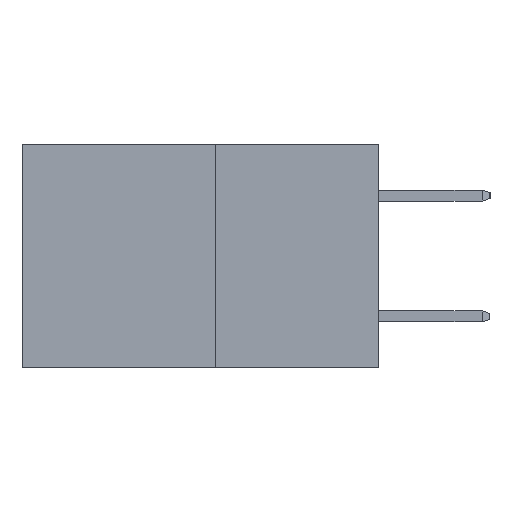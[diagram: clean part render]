
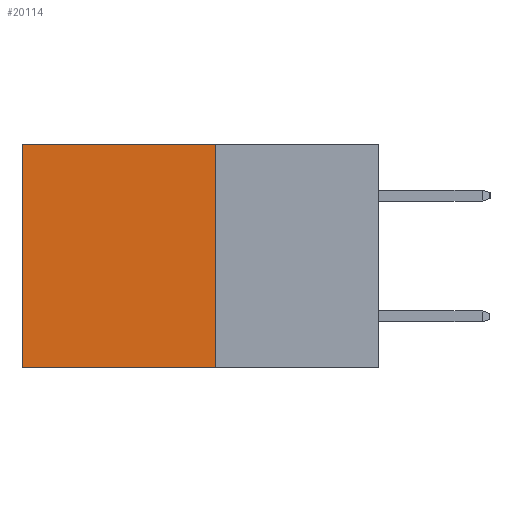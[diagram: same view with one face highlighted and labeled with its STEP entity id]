
A CAD part, left-side view. The second image highlights one B-rep face of the part: STEP entity #20114.
In plain terms, the highlighted planar face has unit normal (-1, 0, 0).
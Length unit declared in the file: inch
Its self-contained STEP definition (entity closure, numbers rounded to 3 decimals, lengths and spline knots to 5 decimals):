
#370 = VECTOR ( 'NONE', #7901, 39.37008 ) ;
#1036 = EDGE_LOOP ( 'NONE', ( #13480, #3146, #9944, #14698 ) ) ;
#1885 = CARTESIAN_POINT ( 'NONE',  ( 0.277, 0.59, -0.37 ) ) ;
#2615 = DIRECTION ( 'NONE',  ( 1., 0., 0. ) ) ;
#3146 = ORIENTED_EDGE ( 'NONE', *, *, #12258, .F. ) ;
#5349 = VERTEX_POINT ( 'NONE', #1885 ) ;
#5377 = LINE ( 'NONE', #17044, #370 ) ;
#5748 = VERTEX_POINT ( 'NONE', #22098 ) ;
#6297 = PLANE ( 'NONE',  #23699 ) ;
#7901 = DIRECTION ( 'NONE',  ( 0., 1., 0. ) ) ;
#8111 = LINE ( 'NONE', #21668, #17305 ) ;
#8784 = CARTESIAN_POINT ( 'NONE',  ( 0.277, 0.27, -0.37 ) ) ;
#8902 = DIRECTION ( 'NONE',  ( 0., 0., -1. ) ) ;
#9064 = VECTOR ( 'NONE', #17220, 39.37008 ) ;
#9944 = ORIENTED_EDGE ( 'NONE', *, *, #23379, .F. ) ;
#10613 = FACE_OUTER_BOUND ( 'NONE', #1036, .T. ) ;
#11585 = DIRECTION ( 'NONE',  ( 0., 0., -1. ) ) ;
#12258 = EDGE_CURVE ( 'NONE', #14520, #5349, #14532, .T. ) ;
#12413 = VERTEX_POINT ( 'NONE', #13936 ) ;
#13480 = ORIENTED_EDGE ( 'NONE', *, *, #14127, .T. ) ;
#13714 = CARTESIAN_POINT ( 'NONE',  ( 0.277, 0.27, -0.37 ) ) ;
#13936 = CARTESIAN_POINT ( 'NONE',  ( 0.277, 0.27, 0. ) ) ;
#14127 = EDGE_CURVE ( 'NONE', #5748, #5349, #21295, .T. ) ;
#14520 = VERTEX_POINT ( 'NONE', #8784 ) ;
#14532 = LINE ( 'NONE', #15400, #9064 ) ;
#14698 = ORIENTED_EDGE ( 'NONE', *, *, #18760, .T. ) ;
#15400 = CARTESIAN_POINT ( 'NONE',  ( 0.277, 0.27, -0.37 ) ) ;
#15565 = DIRECTION ( 'NONE',  ( 0., 0., -1. ) ) ;
#16436 = VECTOR ( 'NONE', #11585, 39.37008 ) ;
#17044 = CARTESIAN_POINT ( 'NONE',  ( 0.277, 0.27, 0. ) ) ;
#17220 = DIRECTION ( 'NONE',  ( 0., 1., 0. ) ) ;
#17305 = VECTOR ( 'NONE', #8902, 39.37008 ) ;
#18760 = EDGE_CURVE ( 'NONE', #12413, #5748, #5377, .T. ) ;
#18819 = CARTESIAN_POINT ( 'NONE',  ( 0.277, 0.59, -0.37 ) ) ;
#20114 = ADVANCED_FACE ( 'NONE', ( #10613 ), #6297, .F. ) ;
#21295 = LINE ( 'NONE', #18819, #16436 ) ;
#21668 = CARTESIAN_POINT ( 'NONE',  ( 0.277, 0.27, -0.37 ) ) ;
#22098 = CARTESIAN_POINT ( 'NONE',  ( 0.277, 0.59, 0. ) ) ;
#23379 = EDGE_CURVE ( 'NONE', #12413, #14520, #8111, .T. ) ;
#23699 = AXIS2_PLACEMENT_3D ( 'NONE', #13714, #2615, #15565 ) ;
